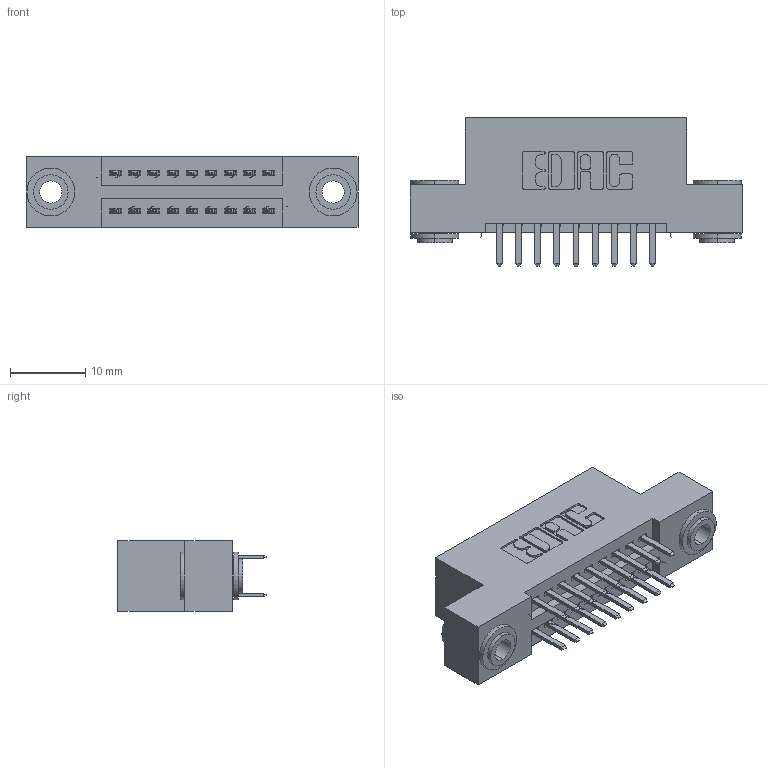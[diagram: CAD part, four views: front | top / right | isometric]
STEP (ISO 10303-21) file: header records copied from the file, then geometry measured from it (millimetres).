
FILE_DESCRIPTION (( 'STEP AP203' ), '1' );
FILE_NAME ('345-018-520-203.STEP', '2018-08-19T05:30:16', ( '' ), ( '' ), 'SwSTEP 2.0', 'SolidWorks 2016', '' );
FILE_SCHEMA (( 'CONFIG_CONTROL_DESIGN' ));
Length unit declared in the file: inch
Products named in the file (4): 345-018-520-203; 345 Part_Flush Mounting Lugs - 0.156 Dia-TH; 345-292-001_345-293-120; 345-250-002_345-250-002-102
Assembly tree (21 placements, depth 2):
  345-018-520-203
    345 Part_Flush Mounting Lugs - 0.156 Dia-TH
    345-292-001_345-293-120  x18
    345-250-002_345-250-002-102  x2
Bounding box: 44.07 x 19.68 x 9.4 mm (x, y, z)
Volume: 3986 mm3; surface area: 5403.9 mm2
Topology: 21 solids, 21 shells, 1136 faces, 3243 edges, 2128 vertices
Faces by surface type: plane 720, cylinder 408, cone 8
Entity records: 12268 total; most frequent: CARTESIAN_POINT 2075, ORIENTED_EDGE 1990, DIRECTION 1889, EDGE_CURVE 995, LINE 799, VECTOR 799, VERTEX_POINT 658, AXIS2_PLACEMENT_3D 545
